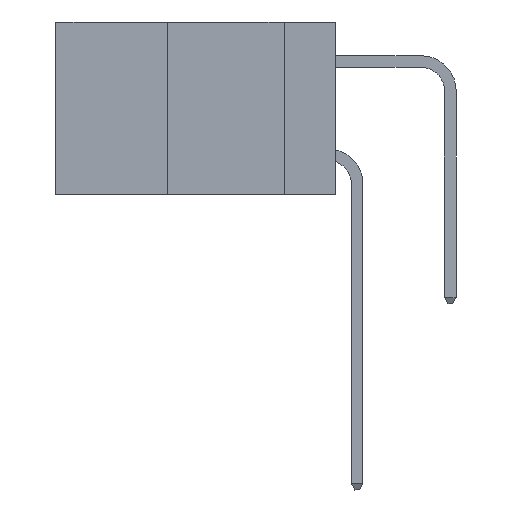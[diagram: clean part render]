
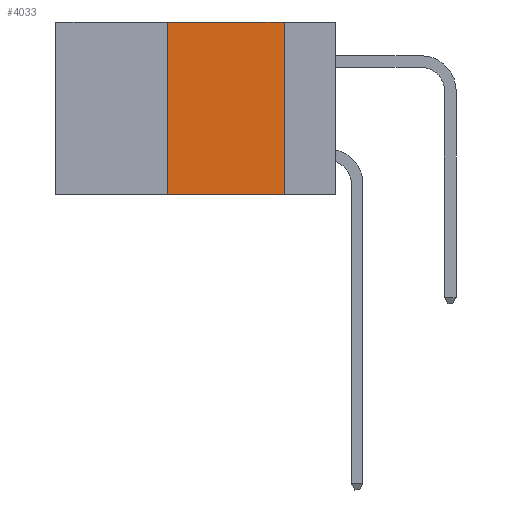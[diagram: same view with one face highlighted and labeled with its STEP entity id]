
A CAD part, left-side view. The second image highlights one B-rep face of the part: STEP entity #4033.
In plain terms, the highlighted planar face has unit normal (-1, 0, 0).
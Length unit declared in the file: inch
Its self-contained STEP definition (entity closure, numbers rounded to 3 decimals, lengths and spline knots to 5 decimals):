
#784 = VECTOR ( 'NONE', #794, 39.37008 ) ;
#794 = DIRECTION ( 'NONE',  ( 0., 0., -1. ) ) ;
#1481 = CARTESIAN_POINT ( 'NONE',  ( 0., 0.36, 0. ) ) ;
#1618 = ORIENTED_EDGE ( 'NONE', *, *, #6249, .F. ) ;
#1786 = ORIENTED_EDGE ( 'NONE', *, *, #2287, .F. ) ;
#2177 = CARTESIAN_POINT ( 'NONE',  ( 0., 0.11, 0. ) ) ;
#2287 = EDGE_CURVE ( 'NONE', #39369, #21708, #28379, .T. ) ;
#2762 = FACE_OUTER_BOUND ( 'NONE', #10606, .T. ) ;
#2920 = PLANE ( 'NONE',  #42390 ) ;
#3515 = VECTOR ( 'NONE', #40847, 39.37008 ) ;
#4033 = ADVANCED_FACE ( 'NONE', ( #2762 ), #2920, .F. ) ;
#4405 = CARTESIAN_POINT ( 'NONE',  ( 0., 0.6, 0. ) ) ;
#6219 = CARTESIAN_POINT ( 'NONE',  ( 0., 0.6, 0. ) ) ;
#6249 = EDGE_CURVE ( 'NONE', #21708, #10877, #12896, .T. ) ;
#8325 = EDGE_CURVE ( 'NONE', #10877, #37017, #11772, .T. ) ;
#10606 = EDGE_LOOP ( 'NONE', ( #16785, #1618, #1786, #39072 ) ) ;
#10609 = CARTESIAN_POINT ( 'NONE',  ( 0., 0.6, -0.37 ) ) ;
#10877 = VERTEX_POINT ( 'NONE', #2177 ) ;
#11772 = LINE ( 'NONE', #20664, #784 ) ;
#12896 = LINE ( 'NONE', #4405, #39593 ) ;
#13112 = CARTESIAN_POINT ( 'NONE',  ( 0., 0.36, 0. ) ) ;
#13125 = VECTOR ( 'NONE', #31541, 39.37008 ) ;
#14021 = CARTESIAN_POINT ( 'NONE',  ( 0., 0.11, -0.37 ) ) ;
#15542 = LINE ( 'NONE', #10609, #3515 ) ;
#16590 = DIRECTION ( 'NONE',  ( 0., 0., -1. ) ) ;
#16785 = ORIENTED_EDGE ( 'NONE', *, *, #8325, .F. ) ;
#17545 = DIRECTION ( 'NONE',  ( 0., -1., 0. ) ) ;
#20664 = CARTESIAN_POINT ( 'NONE',  ( 0., 0.11, 0. ) ) ;
#21708 = VERTEX_POINT ( 'NONE', #13112 ) ;
#28379 = LINE ( 'NONE', #1481, #13125 ) ;
#28537 = EDGE_CURVE ( 'NONE', #39369, #37017, #15542, .T. ) ;
#29079 = CARTESIAN_POINT ( 'NONE',  ( 0., 0.36, -0.37 ) ) ;
#29891 = DIRECTION ( 'NONE',  ( 1., 0., 0. ) ) ;
#31541 = DIRECTION ( 'NONE',  ( 0., 0., 1. ) ) ;
#37017 = VERTEX_POINT ( 'NONE', #14021 ) ;
#39072 = ORIENTED_EDGE ( 'NONE', *, *, #28537, .T. ) ;
#39369 = VERTEX_POINT ( 'NONE', #29079 ) ;
#39593 = VECTOR ( 'NONE', #17545, 39.37008 ) ;
#40847 = DIRECTION ( 'NONE',  ( 0., -1., 0. ) ) ;
#42390 = AXIS2_PLACEMENT_3D ( 'NONE', #6219, #29891, #16590 ) ;
